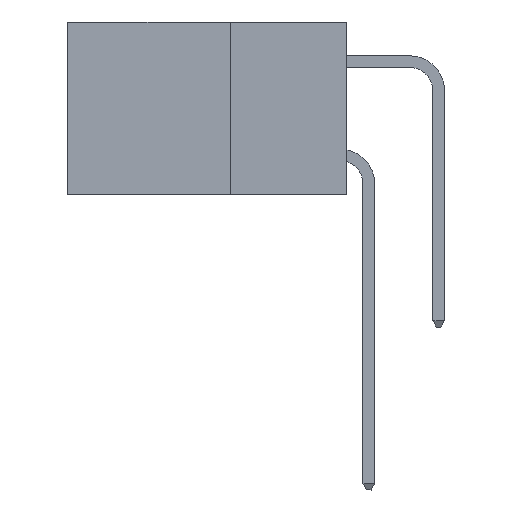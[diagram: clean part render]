
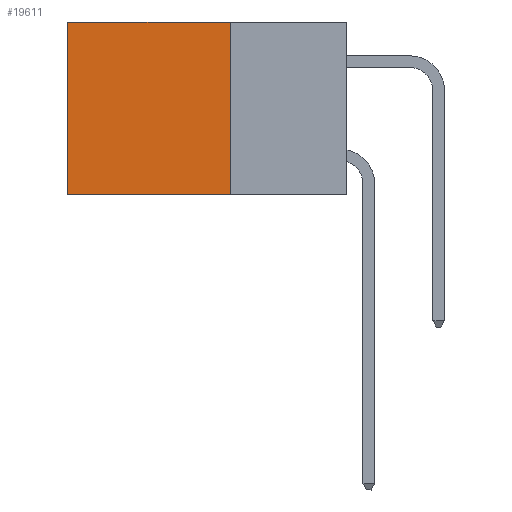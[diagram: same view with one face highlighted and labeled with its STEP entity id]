
A CAD part, left-side view. The second image highlights one B-rep face of the part: STEP entity #19611.
In plain terms, the highlighted planar face has unit normal (-1, 0, 0).
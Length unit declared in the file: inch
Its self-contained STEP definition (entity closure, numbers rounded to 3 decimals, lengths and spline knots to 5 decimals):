
#1282 = CARTESIAN_POINT ( 'NONE',  ( 0.2875, 0.25, 0. ) ) ;
#1358 = ORIENTED_EDGE ( 'NONE', *, *, #13595, .F. ) ;
#1658 = CARTESIAN_POINT ( 'NONE',  ( 0.2875, 0.6, 0. ) ) ;
#3251 = EDGE_CURVE ( 'NONE', #22817, #11465, #7827, .T. ) ;
#4371 = LINE ( 'NONE', #11182, #36297 ) ;
#4603 = EDGE_CURVE ( 'NONE', #25884, #11465, #4371, .T. ) ;
#6470 = DIRECTION ( 'NONE',  ( 0., 1., 0. ) ) ;
#7571 = FACE_OUTER_BOUND ( 'NONE', #38994, .T. ) ;
#7827 = LINE ( 'NONE', #1658, #12341 ) ;
#8477 = DIRECTION ( 'NONE',  ( 0., 0., -1. ) ) ;
#11097 = CARTESIAN_POINT ( 'NONE',  ( 0.2875, 0.6, 0. ) ) ;
#11182 = CARTESIAN_POINT ( 'NONE',  ( 0.2875, 0.25, -0.37 ) ) ;
#11383 = VECTOR ( 'NONE', #31313, 39.37008 ) ;
#11465 = VERTEX_POINT ( 'NONE', #34122 ) ;
#12341 = VECTOR ( 'NONE', #8477, 39.37008 ) ;
#12647 = LINE ( 'NONE', #23187, #27061 ) ;
#13296 = PLANE ( 'NONE',  #17554 ) ;
#13595 = EDGE_CURVE ( 'NONE', #41667, #25884, #37930, .T. ) ;
#17554 = AXIS2_PLACEMENT_3D ( 'NONE', #40635, #20995, #27376 ) ;
#17576 = DIRECTION ( 'NONE',  ( 0., 1., 0. ) ) ;
#18429 = ORIENTED_EDGE ( 'NONE', *, *, #4603, .F. ) ;
#19611 = ADVANCED_FACE ( 'NONE', ( #7571 ), #13296, .F. ) ;
#19679 = ORIENTED_EDGE ( 'NONE', *, *, #3251, .T. ) ;
#20995 = DIRECTION ( 'NONE',  ( 1., 0., 0. ) ) ;
#22817 = VERTEX_POINT ( 'NONE', #11097 ) ;
#23187 = CARTESIAN_POINT ( 'NONE',  ( 0.2875, 0.25, 0. ) ) ;
#25884 = VERTEX_POINT ( 'NONE', #31057 ) ;
#27061 = VECTOR ( 'NONE', #6470, 39.37008 ) ;
#27376 = DIRECTION ( 'NONE',  ( 0., 0., -1. ) ) ;
#31057 = CARTESIAN_POINT ( 'NONE',  ( 0.2875, 0.25, -0.37 ) ) ;
#31313 = DIRECTION ( 'NONE',  ( 0., 0., -1. ) ) ;
#34122 = CARTESIAN_POINT ( 'NONE',  ( 0.2875, 0.6, -0.37 ) ) ;
#34197 = CARTESIAN_POINT ( 'NONE',  ( 0.2875, 0.25, 0. ) ) ;
#34233 = ORIENTED_EDGE ( 'NONE', *, *, #35398, .T. ) ;
#35398 = EDGE_CURVE ( 'NONE', #41667, #22817, #12647, .T. ) ;
#36297 = VECTOR ( 'NONE', #17576, 39.37008 ) ;
#37930 = LINE ( 'NONE', #34197, #11383 ) ;
#38994 = EDGE_LOOP ( 'NONE', ( #19679, #18429, #1358, #34233 ) ) ;
#40635 = CARTESIAN_POINT ( 'NONE',  ( 0.2875, 0.25, 0. ) ) ;
#41667 = VERTEX_POINT ( 'NONE', #1282 ) ;
